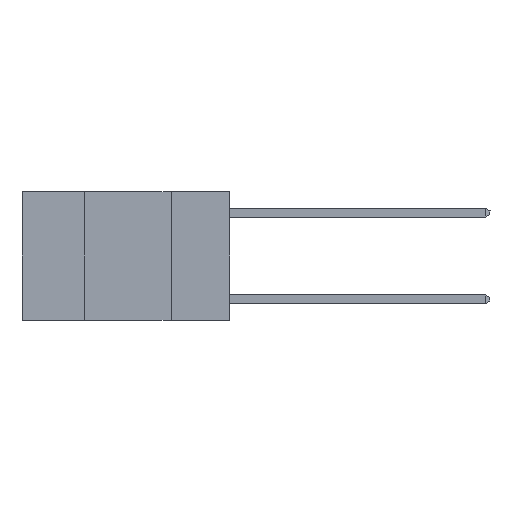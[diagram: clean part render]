
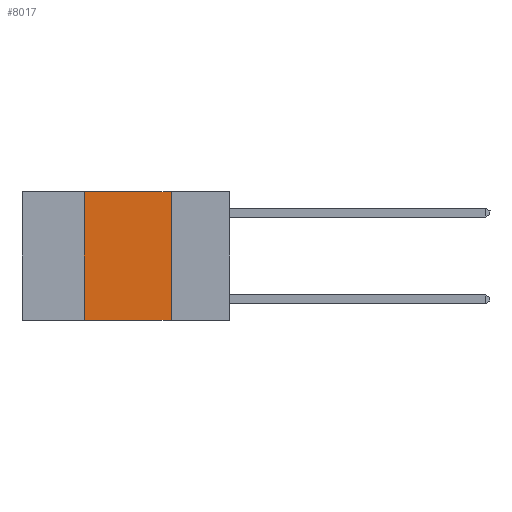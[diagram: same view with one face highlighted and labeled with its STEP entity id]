
A CAD part, left-side view. The second image highlights one B-rep face of the part: STEP entity #8017.
In plain terms, the highlighted planar face has unit normal (-1, 0, 0).
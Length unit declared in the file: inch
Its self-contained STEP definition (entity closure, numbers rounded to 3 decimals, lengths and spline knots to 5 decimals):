
#682 = PLANE ( 'NONE',  #7394 ) ;
#712 = DIRECTION ( 'NONE',  ( 0., -1., 0. ) ) ;
#1194 = CARTESIAN_POINT ( 'NONE',  ( 0., 0.42, 0. ) ) ;
#1348 = ORIENTED_EDGE ( 'NONE', *, *, #6989, .F. ) ;
#1863 = VERTEX_POINT ( 'NONE', #8611 ) ;
#2494 = DIRECTION ( 'NONE',  ( 0., 0., 1. ) ) ;
#2840 = CARTESIAN_POINT ( 'NONE',  ( 0., 0.6, 0. ) ) ;
#3044 = VERTEX_POINT ( 'NONE', #5923 ) ;
#3236 = EDGE_CURVE ( 'NONE', #3044, #3728, #5882, .T. ) ;
#3289 = DIRECTION ( 'NONE',  ( 0., 0., -1. ) ) ;
#3318 = EDGE_LOOP ( 'NONE', ( #6871, #7273, #1348, #7483 ) ) ;
#3367 = VECTOR ( 'NONE', #6975, 39.37008 ) ;
#3428 = DIRECTION ( 'NONE',  ( 0., 0., -1. ) ) ;
#3525 = VECTOR ( 'NONE', #2494, 39.37008 ) ;
#3728 = VERTEX_POINT ( 'NONE', #8155 ) ;
#4073 = LINE ( 'NONE', #1194, #3525 ) ;
#4740 = DIRECTION ( 'NONE',  ( 1., 0., 0. ) ) ;
#4847 = CARTESIAN_POINT ( 'NONE',  ( 0., 0.42, -0.37 ) ) ;
#5357 = VECTOR ( 'NONE', #712, 39.37008 ) ;
#5480 = FACE_OUTER_BOUND ( 'NONE', #3318, .T. ) ;
#5779 = EDGE_CURVE ( 'NONE', #5789, #1863, #6190, .T. ) ;
#5789 = VERTEX_POINT ( 'NONE', #4847 ) ;
#5882 = LINE ( 'NONE', #6635, #5357 ) ;
#5923 = CARTESIAN_POINT ( 'NONE',  ( 0., 0.42, 0. ) ) ;
#6085 = CARTESIAN_POINT ( 'NONE',  ( 0., 0.17, 0. ) ) ;
#6149 = CARTESIAN_POINT ( 'NONE',  ( 0., 0.6, -0.37 ) ) ;
#6190 = LINE ( 'NONE', #6149, #3367 ) ;
#6635 = CARTESIAN_POINT ( 'NONE',  ( 0., 0.6, 0. ) ) ;
#6871 = ORIENTED_EDGE ( 'NONE', *, *, #7328, .F. ) ;
#6975 = DIRECTION ( 'NONE',  ( 0., -1., 0. ) ) ;
#6989 = EDGE_CURVE ( 'NONE', #5789, #3044, #4073, .T. ) ;
#7273 = ORIENTED_EDGE ( 'NONE', *, *, #3236, .F. ) ;
#7286 = LINE ( 'NONE', #6085, #8870 ) ;
#7328 = EDGE_CURVE ( 'NONE', #3728, #1863, #7286, .T. ) ;
#7394 = AXIS2_PLACEMENT_3D ( 'NONE', #2840, #4740, #3428 ) ;
#7483 = ORIENTED_EDGE ( 'NONE', *, *, #5779, .T. ) ;
#8017 = ADVANCED_FACE ( 'NONE', ( #5480 ), #682, .F. ) ;
#8155 = CARTESIAN_POINT ( 'NONE',  ( 0., 0.17, 0. ) ) ;
#8611 = CARTESIAN_POINT ( 'NONE',  ( 0., 0.17, -0.37 ) ) ;
#8870 = VECTOR ( 'NONE', #3289, 39.37008 ) ;
